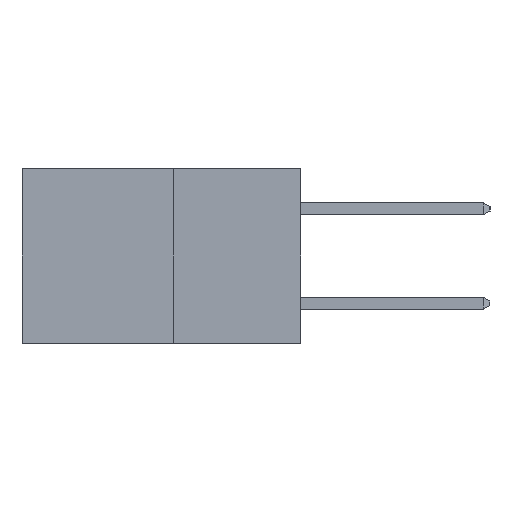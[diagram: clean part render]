
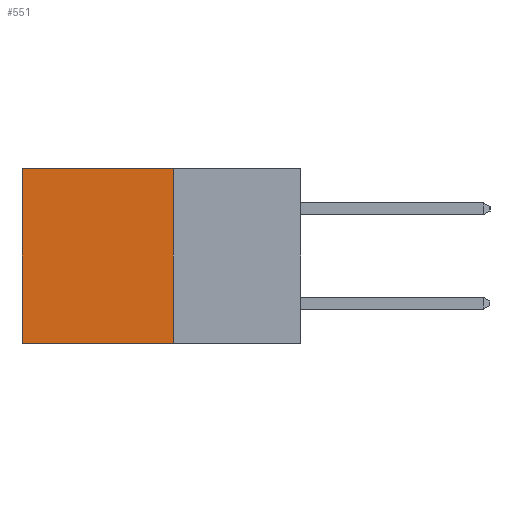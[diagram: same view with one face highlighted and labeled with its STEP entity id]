
A CAD part, left-side view. The second image highlights one B-rep face of the part: STEP entity #551.
In plain terms, the highlighted planar face has unit normal (-1, 0, 0).
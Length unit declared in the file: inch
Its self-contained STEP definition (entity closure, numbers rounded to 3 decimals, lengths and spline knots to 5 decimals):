
#489 = EDGE_CURVE ( 'NONE', #7879, #5440, #2297, .T. ) ;
#494 = EDGE_CURVE ( 'NONE', #7879, #2136, #8177, .T. ) ;
#551 = ADVANCED_FACE ( 'NONE', ( #10063 ), #9523, .F. ) ;
#651 = EDGE_LOOP ( 'NONE', ( #4095, #3355, #2546, #11018 ) ) ;
#1789 = CARTESIAN_POINT ( 'NONE',  ( 0.277, 0.27, -0.37 ) ) ;
#1828 = VERTEX_POINT ( 'NONE', #1931 ) ;
#1931 = CARTESIAN_POINT ( 'NONE',  ( 0.277, 0.59, -0.37 ) ) ;
#1932 = DIRECTION ( 'NONE',  ( 0., 0., -1. ) ) ;
#2136 = VERTEX_POINT ( 'NONE', #3826 ) ;
#2297 = LINE ( 'NONE', #7769, #13579 ) ;
#2546 = ORIENTED_EDGE ( 'NONE', *, *, #489, .F. ) ;
#3355 = ORIENTED_EDGE ( 'NONE', *, *, #6732, .F. ) ;
#3491 = VECTOR ( 'NONE', #5427, 39.37008 ) ;
#3826 = CARTESIAN_POINT ( 'NONE',  ( 0.277, 0.59, 0. ) ) ;
#4095 = ORIENTED_EDGE ( 'NONE', *, *, #12431, .T. ) ;
#5306 = VECTOR ( 'NONE', #8472, 39.37008 ) ;
#5427 = DIRECTION ( 'NONE',  ( 0., 1., 0. ) ) ;
#5440 = VERTEX_POINT ( 'NONE', #5530 ) ;
#5473 = CARTESIAN_POINT ( 'NONE',  ( 0.277, 0.27, -0.37 ) ) ;
#5530 = CARTESIAN_POINT ( 'NONE',  ( 0.277, 0.27, -0.37 ) ) ;
#5980 = DIRECTION ( 'NONE',  ( 0., 0., -1. ) ) ;
#6732 = EDGE_CURVE ( 'NONE', #5440, #1828, #11880, .T. ) ;
#7769 = CARTESIAN_POINT ( 'NONE',  ( 0.277, 0.27, -0.37 ) ) ;
#7879 = VERTEX_POINT ( 'NONE', #10241 ) ;
#8032 = DIRECTION ( 'NONE',  ( 0., 0., -1. ) ) ;
#8177 = LINE ( 'NONE', #9415, #5306 ) ;
#8465 = LINE ( 'NONE', #12483, #10700 ) ;
#8472 = DIRECTION ( 'NONE',  ( 0., 1., 0. ) ) ;
#9415 = CARTESIAN_POINT ( 'NONE',  ( 0.277, 0.27, 0. ) ) ;
#9523 = PLANE ( 'NONE',  #10744 ) ;
#10063 = FACE_OUTER_BOUND ( 'NONE', #651, .T. ) ;
#10241 = CARTESIAN_POINT ( 'NONE',  ( 0.277, 0.27, 0. ) ) ;
#10700 = VECTOR ( 'NONE', #5980, 39.37008 ) ;
#10744 = AXIS2_PLACEMENT_3D ( 'NONE', #1789, #11268, #1932 ) ;
#11018 = ORIENTED_EDGE ( 'NONE', *, *, #494, .T. ) ;
#11268 = DIRECTION ( 'NONE',  ( 1., 0., 0. ) ) ;
#11880 = LINE ( 'NONE', #5473, #3491 ) ;
#12431 = EDGE_CURVE ( 'NONE', #2136, #1828, #8465, .T. ) ;
#12483 = CARTESIAN_POINT ( 'NONE',  ( 0.277, 0.59, -0.37 ) ) ;
#13579 = VECTOR ( 'NONE', #8032, 39.37008 ) ;
